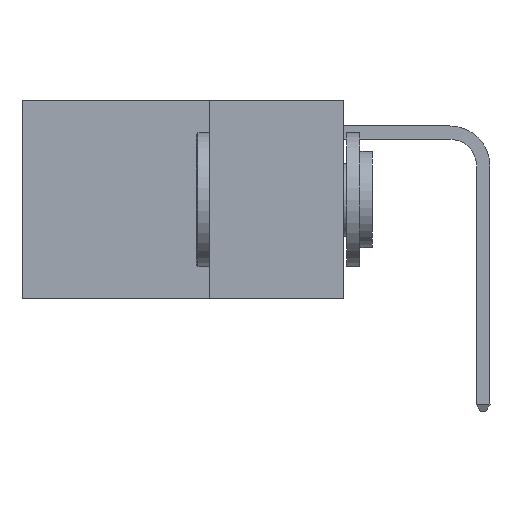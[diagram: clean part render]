
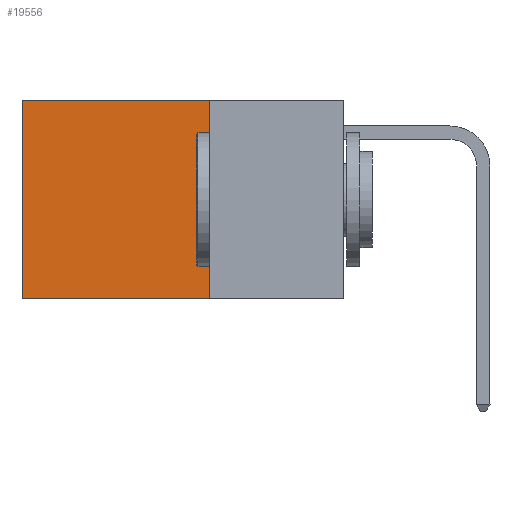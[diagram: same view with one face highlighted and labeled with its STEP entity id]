
A CAD part, left-side view. The second image highlights one B-rep face of the part: STEP entity #19556.
In plain terms, the highlighted planar face has unit normal (-1, 0, 0).
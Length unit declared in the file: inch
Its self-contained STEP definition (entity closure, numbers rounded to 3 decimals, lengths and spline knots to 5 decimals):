
#348 = DIRECTION ( 'NONE',  ( 0., 1., 0. ) ) ;
#1119 = CARTESIAN_POINT ( 'NONE',  ( 0.2625, 0.6, 0. ) ) ;
#2079 = CARTESIAN_POINT ( 'NONE',  ( 0.2625, 0.25, 0. ) ) ;
#3683 = DIRECTION ( 'NONE',  ( 1., 0., 0. ) ) ;
#3975 = VECTOR ( 'NONE', #348, 39.37008 ) ;
#4296 = CARTESIAN_POINT ( 'NONE',  ( 0.2625, 0.25, 0. ) ) ;
#4402 = CARTESIAN_POINT ( 'NONE',  ( 0.2625, 0.25, 0. ) ) ;
#4621 = VERTEX_POINT ( 'NONE', #8398 ) ;
#5322 = DIRECTION ( 'NONE',  ( 0., 0., -1. ) ) ;
#6223 = CARTESIAN_POINT ( 'NONE',  ( 0.2625, 0.6, 0. ) ) ;
#6522 = LINE ( 'NONE', #4402, #3975 ) ;
#6708 = VECTOR ( 'NONE', #14126, 39.37008 ) ;
#6998 = DIRECTION ( 'NONE',  ( 0., 1., 0. ) ) ;
#7897 = DIRECTION ( 'NONE',  ( 0., 0., -1. ) ) ;
#8342 = ORIENTED_EDGE ( 'NONE', *, *, #23770, .F. ) ;
#8398 = CARTESIAN_POINT ( 'NONE',  ( 0.2625, 0.6, -0.37 ) ) ;
#8700 = VERTEX_POINT ( 'NONE', #22465 ) ;
#9361 = EDGE_LOOP ( 'NONE', ( #19314, #8342, #14102, #10400 ) ) ;
#10400 = ORIENTED_EDGE ( 'NONE', *, *, #11690, .T. ) ;
#11690 = EDGE_CURVE ( 'NONE', #24665, #15295, #6522, .T. ) ;
#13768 = LINE ( 'NONE', #4296, #15424 ) ;
#14102 = ORIENTED_EDGE ( 'NONE', *, *, #14924, .F. ) ;
#14126 = DIRECTION ( 'NONE',  ( 0., 0., -1. ) ) ;
#14924 = EDGE_CURVE ( 'NONE', #24665, #8700, #13768, .T. ) ;
#15037 = PLANE ( 'NONE',  #17938 ) ;
#15295 = VERTEX_POINT ( 'NONE', #6223 ) ;
#15424 = VECTOR ( 'NONE', #7897, 39.37008 ) ;
#17938 = AXIS2_PLACEMENT_3D ( 'NONE', #20476, #3683, #5322 ) ;
#18546 = EDGE_CURVE ( 'NONE', #15295, #4621, #20444, .T. ) ;
#18666 = CARTESIAN_POINT ( 'NONE',  ( 0.2625, 0.25, -0.37 ) ) ;
#19314 = ORIENTED_EDGE ( 'NONE', *, *, #18546, .T. ) ;
#19556 = ADVANCED_FACE ( 'NONE', ( #22476 ), #15037, .F. ) ;
#20444 = LINE ( 'NONE', #1119, #6708 ) ;
#20468 = VECTOR ( 'NONE', #6998, 39.37008 ) ;
#20476 = CARTESIAN_POINT ( 'NONE',  ( 0.2625, 0.25, 0. ) ) ;
#20568 = LINE ( 'NONE', #18666, #20468 ) ;
#22465 = CARTESIAN_POINT ( 'NONE',  ( 0.2625, 0.25, -0.37 ) ) ;
#22476 = FACE_OUTER_BOUND ( 'NONE', #9361, .T. ) ;
#23770 = EDGE_CURVE ( 'NONE', #8700, #4621, #20568, .T. ) ;
#24665 = VERTEX_POINT ( 'NONE', #2079 ) ;
